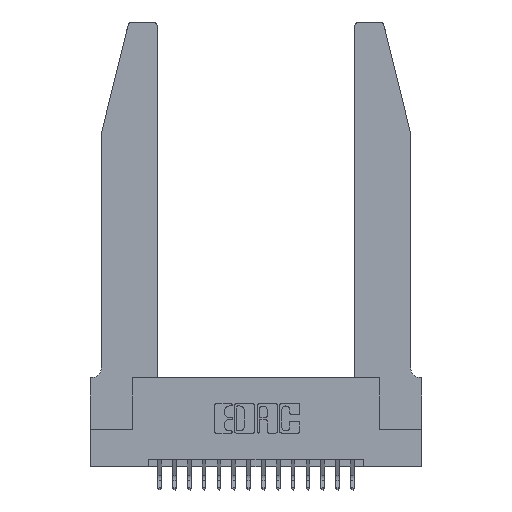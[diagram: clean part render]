
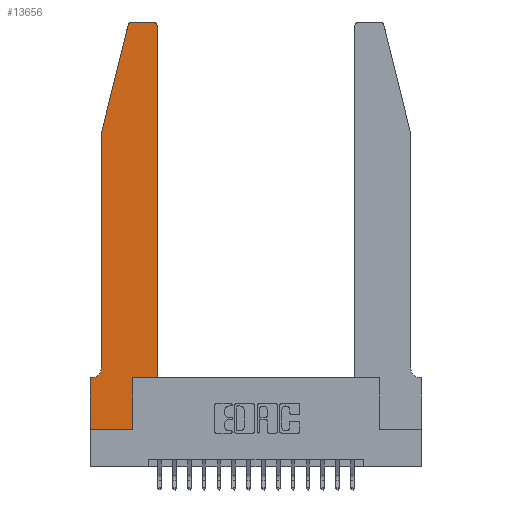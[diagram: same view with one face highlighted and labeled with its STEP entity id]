
A CAD part, top view. The second image highlights one B-rep face of the part: STEP entity #13656.
In plain terms, the highlighted planar face has unit normal (0, 0, 1).
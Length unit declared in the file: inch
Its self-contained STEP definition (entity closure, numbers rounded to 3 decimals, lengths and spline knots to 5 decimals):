
#413 = ORIENTED_EDGE ( 'NONE', *, *, #8003, .T. ) ;
#499 = ORIENTED_EDGE ( 'NONE', *, *, #12279, .T. ) ;
#564 = CARTESIAN_POINT ( 'NONE',  ( 0., 0., 0.37 ) ) ;
#674 = CARTESIAN_POINT ( 'NONE',  ( 0.0055, 0.42, 0.37 ) ) ;
#823 = CARTESIAN_POINT ( 'NONE',  ( 0.0755, 2., 0.37 ) ) ;
#886 = LINE ( 'NONE', #5322, #18762 ) ;
#1081 = LINE ( 'NONE', #8275, #8271 ) ;
#1233 = CARTESIAN_POINT ( 'NONE',  ( 0., 0.35, 0.37 ) ) ;
#1673 = EDGE_CURVE ( 'NONE', #8760, #7914, #11281, .T. ) ;
#1854 = AXIS2_PLACEMENT_3D ( 'NONE', #674, #18712, #3733 ) ;
#1948 = ORIENTED_EDGE ( 'NONE', *, *, #3482, .T. ) ;
#2160 = LINE ( 'NONE', #13777, #19571 ) ;
#2558 = VECTOR ( 'NONE', #14039, 39.37008 ) ;
#2819 = VERTEX_POINT ( 'NONE', #1233 ) ;
#2848 = VECTOR ( 'NONE', #11250, 39.37008 ) ;
#2923 = DIRECTION ( 'NONE',  ( 0., 0., 1. ) ) ;
#3205 = CARTESIAN_POINT ( 'NONE',  ( 0.0755, 0.42, 0.37 ) ) ;
#3363 = PLANE ( 'NONE',  #11248 ) ;
#3375 = VERTEX_POINT ( 'NONE', #3205 ) ;
#3482 = EDGE_CURVE ( 'NONE', #2819, #18296, #12558, .T. ) ;
#3497 = CARTESIAN_POINT ( 'NONE',  ( 0.2865, 0.35, 0.37 ) ) ;
#3517 = CARTESIAN_POINT ( 'NONE',  ( 0., 0., 0.37 ) ) ;
#3723 = VERTEX_POINT ( 'NONE', #16339 ) ;
#3733 = DIRECTION ( 'NONE',  ( -1., 0., 0. ) ) ;
#4126 = VERTEX_POINT ( 'NONE', #19425 ) ;
#4347 = ORIENTED_EDGE ( 'NONE', *, *, #1673, .T. ) ;
#5322 = CARTESIAN_POINT ( 'NONE',  ( 0.0755, 0.35, 0.37 ) ) ;
#5701 = EDGE_CURVE ( 'NONE', #3723, #4126, #9647, .T. ) ;
#5819 = CARTESIAN_POINT ( 'NONE',  ( 0.4505, 0.35, 0.37 ) ) ;
#5875 = CARTESIAN_POINT ( 'NONE',  ( 0.25487, 2.72718, 0.37 ) ) ;
#5927 = VECTOR ( 'NONE', #14798, 39.37008 ) ;
#5954 = DIRECTION ( 'NONE',  ( 0., 0., 1. ) ) ;
#6321 = CARTESIAN_POINT ( 'NONE',  ( 0., 0.35, 0.37 ) ) ;
#6387 = DIRECTION ( 'NONE',  ( 1., 0., 0. ) ) ;
#6654 = ORIENTED_EDGE ( 'NONE', *, *, #9682, .T. ) ;
#7188 = DIRECTION ( 'NONE',  ( -1., 0., 0. ) ) ;
#7548 = EDGE_CURVE ( 'NONE', #7914, #9328, #9334, .T. ) ;
#7855 = EDGE_CURVE ( 'NONE', #9328, #17068, #12663, .T. ) ;
#7914 = VERTEX_POINT ( 'NONE', #14463 ) ;
#8003 = EDGE_CURVE ( 'NONE', #10968, #3723, #2160, .T. ) ;
#8271 = VECTOR ( 'NONE', #17541, 39.37008 ) ;
#8275 = CARTESIAN_POINT ( 'NONE',  ( 0.0755, 2., 0.37 ) ) ;
#8760 = VERTEX_POINT ( 'NONE', #17100 ) ;
#8865 = EDGE_CURVE ( 'NONE', #18296, #17539, #19310, .T. ) ;
#8871 = CARTESIAN_POINT ( 'NONE',  ( 0.0755, 2., 0.37 ) ) ;
#9000 = ORIENTED_EDGE ( 'NONE', *, *, #12044, .T. ) ;
#9328 = VERTEX_POINT ( 'NONE', #5875 ) ;
#9334 = CIRCLE ( 'NONE', #16511, 0.03 ) ;
#9559 = ORIENTED_EDGE ( 'NONE', *, *, #17451, .T. ) ;
#9647 = LINE ( 'NONE', #5819, #10615 ) ;
#9682 = EDGE_CURVE ( 'NONE', #17068, #3375, #1081, .T. ) ;
#9865 = CARTESIAN_POINT ( 'NONE',  ( 0.2865, 0., 0.37 ) ) ;
#10501 = CARTESIAN_POINT ( 'NONE',  ( 0., 0., 0.37 ) ) ;
#10591 = CIRCLE ( 'NONE', #17976, 0.03 ) ;
#10615 = VECTOR ( 'NONE', #19396, 39.37008 ) ;
#10784 = VECTOR ( 'NONE', #19008, 39.37008 ) ;
#10968 = VERTEX_POINT ( 'NONE', #3497 ) ;
#11248 = AXIS2_PLACEMENT_3D ( 'NONE', #6321, #12030, #6387 ) ;
#11250 = DIRECTION ( 'NONE',  ( 1., 0., 0. ) ) ;
#11281 = LINE ( 'NONE', #14886, #14589 ) ;
#12030 = DIRECTION ( 'NONE',  ( 0., 0., 1. ) ) ;
#12042 = CARTESIAN_POINT ( 'NONE',  ( 0.284, 2.72, 0.37 ) ) ;
#12044 = EDGE_CURVE ( 'NONE', #4126, #8760, #10591, .T. ) ;
#12218 = CIRCLE ( 'NONE', #1854, 0.07 ) ;
#12279 = EDGE_CURVE ( 'NONE', #3375, #18396, #12218, .T. ) ;
#12558 = LINE ( 'NONE', #3517, #2558 ) ;
#12621 = ORIENTED_EDGE ( 'NONE', *, *, #7548, .T. ) ;
#12663 = LINE ( 'NONE', #823, #10784 ) ;
#13570 = DIRECTION ( 'NONE',  ( 1., 0., 0. ) ) ;
#13656 = ADVANCED_FACE ( 'NONE', ( #15267 ), #3363, .T. ) ;
#13777 = CARTESIAN_POINT ( 'NONE',  ( 0.4505, 0.35, 0.37 ) ) ;
#14039 = DIRECTION ( 'NONE',  ( 0., -1., 0. ) ) ;
#14463 = CARTESIAN_POINT ( 'NONE',  ( 0.284, 2.75, 0.37 ) ) ;
#14589 = VECTOR ( 'NONE', #7188, 39.37008 ) ;
#14798 = DIRECTION ( 'NONE',  ( 0., 1., 0. ) ) ;
#14886 = CARTESIAN_POINT ( 'NONE',  ( 0.2605, 2.75, 0.37 ) ) ;
#15069 = CARTESIAN_POINT ( 'NONE',  ( 0.4205, 2.72, 0.37 ) ) ;
#15267 = FACE_OUTER_BOUND ( 'NONE', #17443, .T. ) ;
#15465 = DIRECTION ( 'NONE',  ( 1., 0., 0. ) ) ;
#16260 = ORIENTED_EDGE ( 'NONE', *, *, #7855, .T. ) ;
#16331 = EDGE_CURVE ( 'NONE', #17539, #10968, #17863, .T. ) ;
#16339 = CARTESIAN_POINT ( 'NONE',  ( 0.4505, 0.35, 0.37 ) ) ;
#16511 = AXIS2_PLACEMENT_3D ( 'NONE', #12042, #2923, #13570 ) ;
#17068 = VERTEX_POINT ( 'NONE', #8871 ) ;
#17100 = CARTESIAN_POINT ( 'NONE',  ( 0.4205, 2.75, 0.37 ) ) ;
#17443 = EDGE_LOOP ( 'NONE', ( #4347, #12621, #16260, #6654, #499, #9559, #1948, #18122, #18062, #413, #19666, #9000 ) ) ;
#17451 = EDGE_CURVE ( 'NONE', #18396, #2819, #886, .T. ) ;
#17539 = VERTEX_POINT ( 'NONE', #9865 ) ;
#17541 = DIRECTION ( 'NONE',  ( 0., -1., 0. ) ) ;
#17863 = LINE ( 'NONE', #19147, #5927 ) ;
#17976 = AXIS2_PLACEMENT_3D ( 'NONE', #15069, #5954, #19657 ) ;
#18062 = ORIENTED_EDGE ( 'NONE', *, *, #16331, .T. ) ;
#18122 = ORIENTED_EDGE ( 'NONE', *, *, #8865, .T. ) ;
#18296 = VERTEX_POINT ( 'NONE', #10501 ) ;
#18396 = VERTEX_POINT ( 'NONE', #18676 ) ;
#18676 = CARTESIAN_POINT ( 'NONE',  ( 0.0055, 0.35, 0.37 ) ) ;
#18712 = DIRECTION ( 'NONE',  ( 0., 0., -1. ) ) ;
#18762 = VECTOR ( 'NONE', #18899, 39.37008 ) ;
#18899 = DIRECTION ( 'NONE',  ( -1., 0., 0. ) ) ;
#19008 = DIRECTION ( 'NONE',  ( -0.239, -0.971, 0. ) ) ;
#19147 = CARTESIAN_POINT ( 'NONE',  ( 0.2865, 0.35, 0.37 ) ) ;
#19310 = LINE ( 'NONE', #564, #2848 ) ;
#19396 = DIRECTION ( 'NONE',  ( 0., 1., 0. ) ) ;
#19425 = CARTESIAN_POINT ( 'NONE',  ( 0.4505, 2.72, 0.37 ) ) ;
#19571 = VECTOR ( 'NONE', #15465, 39.37008 ) ;
#19657 = DIRECTION ( 'NONE',  ( 1., 0., 0. ) ) ;
#19666 = ORIENTED_EDGE ( 'NONE', *, *, #5701, .T. ) ;
